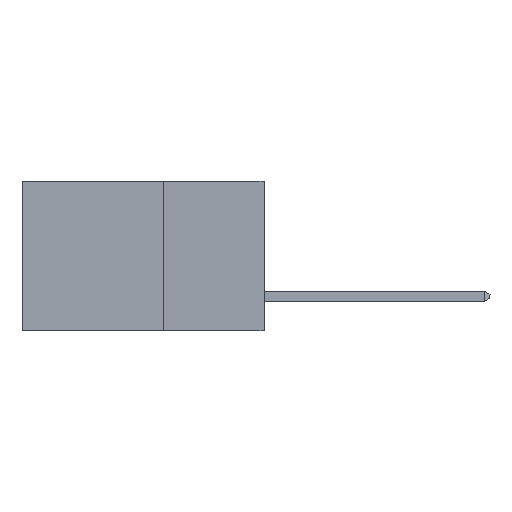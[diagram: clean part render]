
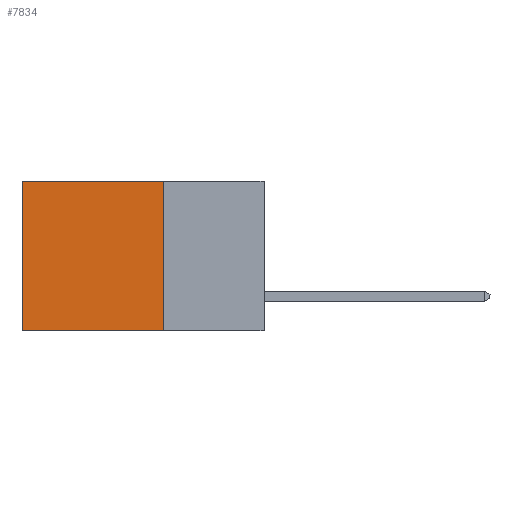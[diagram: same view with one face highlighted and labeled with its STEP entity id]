
A CAD part, left-side view. The second image highlights one B-rep face of the part: STEP entity #7834.
In plain terms, the highlighted planar face has unit normal (-1, 0, 0).
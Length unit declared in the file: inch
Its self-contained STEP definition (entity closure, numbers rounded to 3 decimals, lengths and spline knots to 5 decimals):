
#111 = VERTEX_POINT ( 'NONE', #4288 ) ;
#297 = EDGE_CURVE ( 'NONE', #1198, #8154, #2642, .T. ) ;
#322 = ORIENTED_EDGE ( 'NONE', *, *, #1181, .T. ) ;
#427 = VECTOR ( 'NONE', #4667, 39.37008 ) ;
#1181 = EDGE_CURVE ( 'NONE', #8154, #111, #1802, .T. ) ;
#1198 = VERTEX_POINT ( 'NONE', #8237 ) ;
#1354 = VERTEX_POINT ( 'NONE', #5513 ) ;
#1802 = LINE ( 'NONE', #3135, #5240 ) ;
#1847 = ORIENTED_EDGE ( 'NONE', *, *, #7618, .F. ) ;
#1956 = DIRECTION ( 'NONE',  ( 1., 0., 0. ) ) ;
#2642 = LINE ( 'NONE', #5499, #427 ) ;
#3135 = CARTESIAN_POINT ( 'NONE',  ( 0.2615, 0.6, -0.37 ) ) ;
#3646 = CARTESIAN_POINT ( 'NONE',  ( 0.2615, 0.25, -0.37 ) ) ;
#3712 = ORIENTED_EDGE ( 'NONE', *, *, #6321, .F. ) ;
#3741 = VECTOR ( 'NONE', #5268, 39.37008 ) ;
#4035 = DIRECTION ( 'NONE',  ( 0., 1., 0. ) ) ;
#4288 = CARTESIAN_POINT ( 'NONE',  ( 0.2615, 0.6, -0.37 ) ) ;
#4635 = VECTOR ( 'NONE', #4035, 39.37008 ) ;
#4667 = DIRECTION ( 'NONE',  ( 0., 1., 0. ) ) ;
#5240 = VECTOR ( 'NONE', #6890, 39.37008 ) ;
#5268 = DIRECTION ( 'NONE',  ( 0., 0., -1. ) ) ;
#5440 = LINE ( 'NONE', #8970, #4635 ) ;
#5499 = CARTESIAN_POINT ( 'NONE',  ( 0.2615, 0.25, 0. ) ) ;
#5513 = CARTESIAN_POINT ( 'NONE',  ( 0.2615, 0.25, -0.37 ) ) ;
#6275 = AXIS2_PLACEMENT_3D ( 'NONE', #3646, #1956, #7484 ) ;
#6321 = EDGE_CURVE ( 'NONE', #1198, #1354, #7288, .T. ) ;
#6890 = DIRECTION ( 'NONE',  ( 0., 0., -1. ) ) ;
#7019 = EDGE_LOOP ( 'NONE', ( #322, #1847, #3712, #8414 ) ) ;
#7219 = PLANE ( 'NONE',  #6275 ) ;
#7288 = LINE ( 'NONE', #8887, #3741 ) ;
#7484 = DIRECTION ( 'NONE',  ( 0., 0., -1. ) ) ;
#7618 = EDGE_CURVE ( 'NONE', #1354, #111, #5440, .T. ) ;
#7834 = ADVANCED_FACE ( 'NONE', ( #8395 ), #7219, .F. ) ;
#8154 = VERTEX_POINT ( 'NONE', #9272 ) ;
#8237 = CARTESIAN_POINT ( 'NONE',  ( 0.2615, 0.25, 0. ) ) ;
#8395 = FACE_OUTER_BOUND ( 'NONE', #7019, .T. ) ;
#8414 = ORIENTED_EDGE ( 'NONE', *, *, #297, .T. ) ;
#8887 = CARTESIAN_POINT ( 'NONE',  ( 0.2615, 0.25, -0.37 ) ) ;
#8970 = CARTESIAN_POINT ( 'NONE',  ( 0.2615, 0.25, -0.37 ) ) ;
#9272 = CARTESIAN_POINT ( 'NONE',  ( 0.2615, 0.6, 0. ) ) ;
